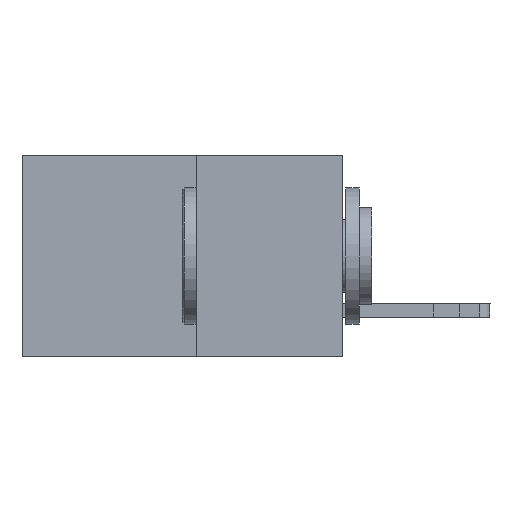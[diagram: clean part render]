
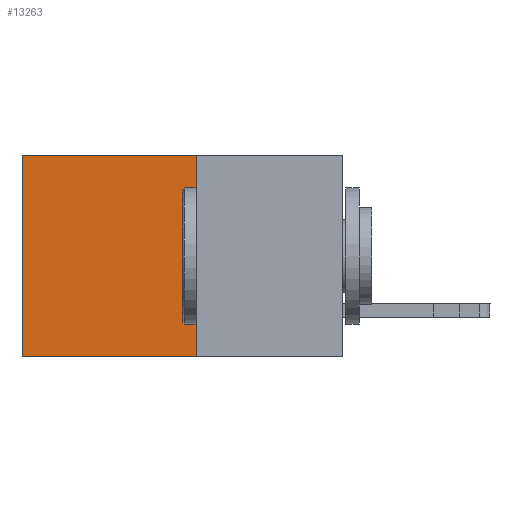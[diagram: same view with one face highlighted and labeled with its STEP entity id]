
A CAD part, left-side view. The second image highlights one B-rep face of the part: STEP entity #13263.
In plain terms, the highlighted planar face has unit normal (-1, 0, 0).
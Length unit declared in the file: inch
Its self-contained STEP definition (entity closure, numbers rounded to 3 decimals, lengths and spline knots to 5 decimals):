
#649 = CARTESIAN_POINT ( 'NONE',  ( 0.277, 0.27, -0.37 ) ) ;
#786 = VERTEX_POINT ( 'NONE', #22271 ) ;
#1710 = VECTOR ( 'NONE', #17713, 39.37008 ) ;
#2315 = CARTESIAN_POINT ( 'NONE',  ( 0.277, 0.59, 0. ) ) ;
#2718 = DIRECTION ( 'NONE',  ( 0., 0., -1. ) ) ;
#3340 = CARTESIAN_POINT ( 'NONE',  ( 0.277, 0.59, -0.37 ) ) ;
#3437 = ORIENTED_EDGE ( 'NONE', *, *, #25484, .F. ) ;
#4014 = ORIENTED_EDGE ( 'NONE', *, *, #7365, .T. ) ;
#4777 = VERTEX_POINT ( 'NONE', #27084 ) ;
#6611 = VECTOR ( 'NONE', #2718, 39.37008 ) ;
#6936 = VECTOR ( 'NONE', #20344, 39.37008 ) ;
#7365 = EDGE_CURVE ( 'NONE', #26598, #9707, #18137, .T. ) ;
#7464 = LINE ( 'NONE', #15538, #1710 ) ;
#7622 = CARTESIAN_POINT ( 'NONE',  ( 0.277, 0.27, -0.37 ) ) ;
#9283 = VECTOR ( 'NONE', #15785, 39.37008 ) ;
#9707 = VERTEX_POINT ( 'NONE', #3340 ) ;
#9823 = DIRECTION ( 'NONE',  ( 0., 0., -1. ) ) ;
#13263 = ADVANCED_FACE ( 'NONE', ( #25977 ), #18396, .F. ) ;
#13536 = CARTESIAN_POINT ( 'NONE',  ( 0.277, 0.59, -0.37 ) ) ;
#14432 = EDGE_CURVE ( 'NONE', #4777, #26598, #17785, .T. ) ;
#15537 = EDGE_CURVE ( 'NONE', #4777, #786, #24484, .T. ) ;
#15538 = CARTESIAN_POINT ( 'NONE',  ( 0.277, 0.27, -0.37 ) ) ;
#15785 = DIRECTION ( 'NONE',  ( 0., 0., -1. ) ) ;
#17713 = DIRECTION ( 'NONE',  ( 0., 1., 0. ) ) ;
#17785 = LINE ( 'NONE', #26807, #6936 ) ;
#18137 = LINE ( 'NONE', #13536, #6611 ) ;
#18396 = PLANE ( 'NONE',  #20546 ) ;
#20344 = DIRECTION ( 'NONE',  ( 0., 1., 0. ) ) ;
#20546 = AXIS2_PLACEMENT_3D ( 'NONE', #7622, #22772, #9823 ) ;
#21161 = EDGE_LOOP ( 'NONE', ( #4014, #3437, #21640, #27213 ) ) ;
#21640 = ORIENTED_EDGE ( 'NONE', *, *, #15537, .F. ) ;
#22271 = CARTESIAN_POINT ( 'NONE',  ( 0.277, 0.27, -0.37 ) ) ;
#22772 = DIRECTION ( 'NONE',  ( 1., 0., 0. ) ) ;
#24484 = LINE ( 'NONE', #649, #9283 ) ;
#25484 = EDGE_CURVE ( 'NONE', #786, #9707, #7464, .T. ) ;
#25977 = FACE_OUTER_BOUND ( 'NONE', #21161, .T. ) ;
#26598 = VERTEX_POINT ( 'NONE', #2315 ) ;
#26807 = CARTESIAN_POINT ( 'NONE',  ( 0.277, 0.27, 0. ) ) ;
#27084 = CARTESIAN_POINT ( 'NONE',  ( 0.277, 0.27, 0. ) ) ;
#27213 = ORIENTED_EDGE ( 'NONE', *, *, #14432, .T. ) ;
